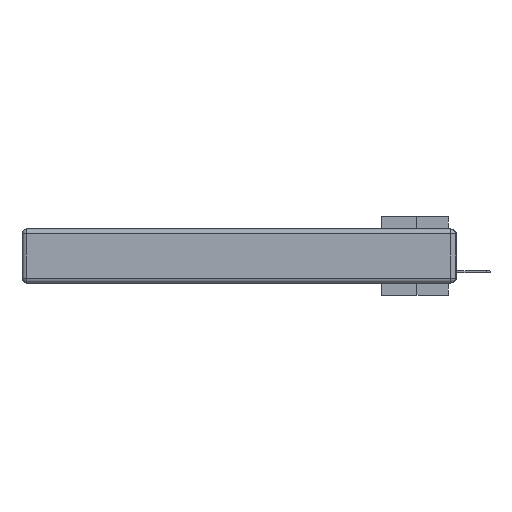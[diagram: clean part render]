
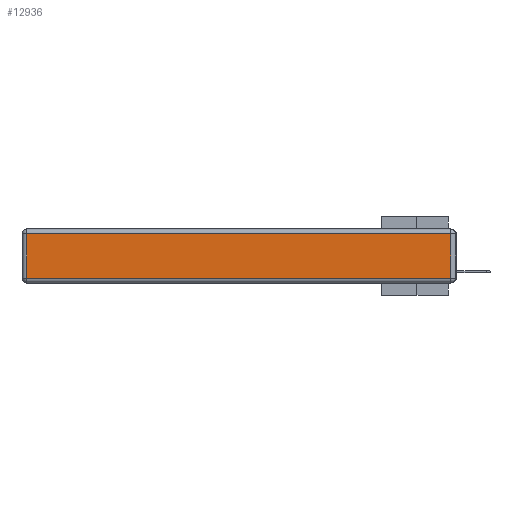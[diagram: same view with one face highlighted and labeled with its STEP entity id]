
A CAD part, left-side view. The second image highlights one B-rep face of the part: STEP entity #12936.
In plain terms, the highlighted planar face has unit normal (-1, 0, 0).
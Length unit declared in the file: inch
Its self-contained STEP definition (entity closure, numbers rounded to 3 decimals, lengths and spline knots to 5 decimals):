
#1296 = DIRECTION ( 'NONE',  ( 0., -1., 0. ) ) ;
#1609 = LINE ( 'NONE', #6001, #16666 ) ;
#2347 = CARTESIAN_POINT ( 'NONE',  ( 0., 2.75, -0.03 ) ) ;
#3017 = ORIENTED_EDGE ( 'NONE', *, *, #12278, .T. ) ;
#3477 = VECTOR ( 'NONE', #3825, 39.37008 ) ;
#3661 = LINE ( 'NONE', #9009, #3477 ) ;
#3741 = DIRECTION ( 'NONE',  ( 0., 0., 1. ) ) ;
#3825 = DIRECTION ( 'NONE',  ( 0., 0., -1. ) ) ;
#4212 = CARTESIAN_POINT ( 'NONE',  ( 0., 2.72, -0.03 ) ) ;
#4327 = EDGE_CURVE ( 'NONE', #24933, #26334, #1609, .T. ) ;
#5867 = DIRECTION ( 'NONE',  ( -1., 0., 0. ) ) ;
#6001 = CARTESIAN_POINT ( 'NONE',  ( 0., 0., -0.313 ) ) ;
#7365 = DIRECTION ( 'NONE',  ( 0., 0., 1. ) ) ;
#7372 = DIRECTION ( 'NONE',  ( 0., 1., 0. ) ) ;
#8406 = VERTEX_POINT ( 'NONE', #4212 ) ;
#8443 = ORIENTED_EDGE ( 'NONE', *, *, #4327, .T. ) ;
#8925 = CARTESIAN_POINT ( 'NONE',  ( 0., 0., -0.343 ) ) ;
#9009 = CARTESIAN_POINT ( 'NONE',  ( 0., 2.72, -0.343 ) ) ;
#10502 = VECTOR ( 'NONE', #7365, 39.37008 ) ;
#10884 = PLANE ( 'NONE',  #24034 ) ;
#11810 = CARTESIAN_POINT ( 'NONE',  ( 0., 2.72, -0.313 ) ) ;
#12278 = EDGE_CURVE ( 'NONE', #26334, #14938, #14537, .T. ) ;
#12526 = ORIENTED_EDGE ( 'NONE', *, *, #13562, .T. ) ;
#12936 = ADVANCED_FACE ( 'NONE', ( #21314 ), #10884, .T. ) ;
#13562 = EDGE_CURVE ( 'NONE', #14938, #8406, #24651, .T. ) ;
#14210 = VECTOR ( 'NONE', #7372, 39.37008 ) ;
#14537 = LINE ( 'NONE', #22043, #10502 ) ;
#14938 = VERTEX_POINT ( 'NONE', #25177 ) ;
#16666 = VECTOR ( 'NONE', #1296, 39.37008 ) ;
#17684 = CARTESIAN_POINT ( 'NONE',  ( 0., 0.03, -0.313 ) ) ;
#18003 = ORIENTED_EDGE ( 'NONE', *, *, #23974, .T. ) ;
#21314 = FACE_OUTER_BOUND ( 'NONE', #29818, .T. ) ;
#22043 = CARTESIAN_POINT ( 'NONE',  ( 0., 0.03, -0.343 ) ) ;
#23974 = EDGE_CURVE ( 'NONE', #8406, #24933, #3661, .T. ) ;
#24034 = AXIS2_PLACEMENT_3D ( 'NONE', #8925, #5867, #3741 ) ;
#24651 = LINE ( 'NONE', #2347, #14210 ) ;
#24933 = VERTEX_POINT ( 'NONE', #11810 ) ;
#25177 = CARTESIAN_POINT ( 'NONE',  ( 0., 0.03, -0.03 ) ) ;
#26334 = VERTEX_POINT ( 'NONE', #17684 ) ;
#29818 = EDGE_LOOP ( 'NONE', ( #8443, #3017, #12526, #18003 ) ) ;
